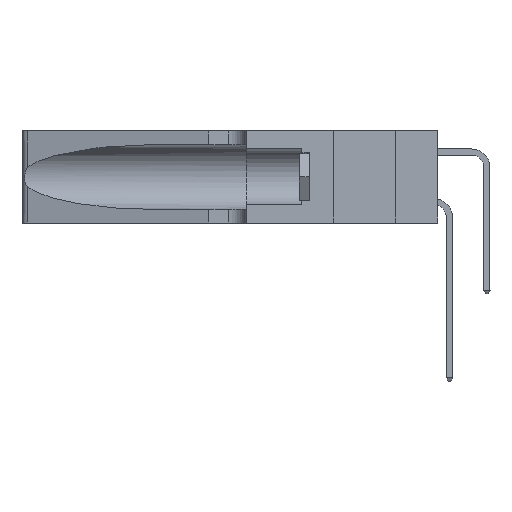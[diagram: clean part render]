
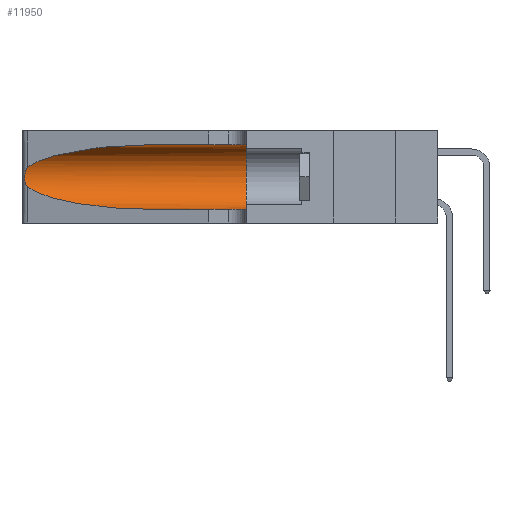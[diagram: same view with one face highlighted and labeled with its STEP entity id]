
A CAD part, left-side view. The second image highlights one B-rep face of the part: STEP entity #11950.
In plain terms, the highlighted cylindrical face has radius 3.308 mm (diameter 6.617 mm), a partial arc.
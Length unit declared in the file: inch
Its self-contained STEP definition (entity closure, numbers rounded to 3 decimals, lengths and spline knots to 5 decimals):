
#690 = CYLINDRICAL_SURFACE ( 'NONE', #15698, 0.13025 ) ;
#820 = CARTESIAN_POINT ( 'NONE',  ( 0.1305, 0.72297, 0.05475 ) ) ;
#1220 = CARTESIAN_POINT ( 'NONE',  ( 0.18966, 0.96281, 0.31525 ) ) ;
#1395 = CARTESIAN_POINT ( 'NONE',  ( 0.25487, 1.22718, 0.22369 ) ) ;
#1634 = EDGE_CURVE ( 'NONE', #3769, #15710, #14663, .T. ) ;
#1723 = CARTESIAN_POINT ( 'NONE',  ( 0.25487, 1.22718, 0.14631 ) ) ;
#2244 = CARTESIAN_POINT ( 'NONE',  ( 0.18966, 0.96281, 0.05475 ) ) ;
#3010 = CARTESIAN_POINT ( 'NONE',  ( 0.26018, 1.23835, 0.19895 ) ) ;
#3198 = CARTESIAN_POINT ( 'NONE',  ( 0.1305, 0.72297, 0.31525 ) ) ;
#3457 = ORIENTED_EDGE ( 'NONE', *, *, #22702, .T. ) ;
#3769 = VERTEX_POINT ( 'NONE', #3198 ) ;
#4048 = CARTESIAN_POINT ( 'NONE',  ( 0.25487, 1.22718, 0.22369 ) ) ;
#4293 = EDGE_LOOP ( 'NONE', ( #13909, #17059, #26115, #3457, #21462, #16241 ) ) ;
#4567 = DIRECTION ( 'NONE',  ( 0., -1., 0. ) ) ;
#5808 = CARTESIAN_POINT ( 'NONE',  ( 0.2373, 1.15595, 0.08982 ) ) ;
#5863 = VERTEX_POINT ( 'NONE', #820 ) ;
#6558 =( BOUNDED_CURVE ( )  B_SPLINE_CURVE ( 3, ( #1723, #5808, #2244, #16350 ),
 .UNSPECIFIED., .F., .F. ) 
 B_SPLINE_CURVE_WITH_KNOTS ( ( 4, 4 ),
 ( 3.44316, 4.71239 ),
 .UNSPECIFIED. ) 
 CURVE ( )  GEOMETRIC_REPRESENTATION_ITEM ( )  RATIONAL_B_SPLINE_CURVE ( ( 1., 0.87, 0.87, 1. ) ) 
 REPRESENTATION_ITEM ( '' )  );
#7334 = CIRCLE ( 'NONE', #14410, 0.13025 ) ;
#7349 = DIRECTION ( 'NONE',  ( 0., 0., 1. ) ) ;
#7541 = CARTESIAN_POINT ( 'NONE',  ( 0.25487, 1.22718, 0.14631 ) ) ;
#9154 = CARTESIAN_POINT ( 'NONE',  ( 0.26017, 1.23833, 0.17102 ) ) ;
#9344 = CARTESIAN_POINT ( 'NONE',  ( 0.26075, 1.23896, 0.19203 ) ) ;
#9787 = DIRECTION ( 'NONE',  ( 0., -1., 0. ) ) ;
#10093 = EDGE_CURVE ( 'NONE', #3769, #18203, #12030, .T. ) ;
#10714 = VERTEX_POINT ( 'NONE', #24264 ) ;
#11950 = ADVANCED_FACE ( 'NONE', ( #21880 ), #690, .F. ) ;
#12030 = LINE ( 'NONE', #18358, #20986 ) ;
#12247 = DIRECTION ( 'NONE',  ( 0., -1., 0. ) ) ;
#13439 = CARTESIAN_POINT ( 'NONE',  ( 0.1305, 0.35, 0.185 ) ) ;
#13536 = EDGE_CURVE ( 'NONE', #15710, #10714, #17473, .T. ) ;
#13671 = CARTESIAN_POINT ( 'NONE',  ( 0.25487, 1.22718, 0.22369 ) ) ;
#13806 = CARTESIAN_POINT ( 'NONE',  ( 0.25789, 1.23486, 0.15765 ) ) ;
#13909 = ORIENTED_EDGE ( 'NONE', *, *, #1634, .T. ) ;
#14410 = AXIS2_PLACEMENT_3D ( 'NONE', #13439, #23691, #7349 ) ;
#14488 = CARTESIAN_POINT ( 'NONE',  ( 0.1305, 1.61858, 0.185 ) ) ;
#14663 =( BOUNDED_CURVE ( )  B_SPLINE_CURVE ( 3, ( #19522, #1220, #19618, #1395 ),
 .UNSPECIFIED., .F., .T. ) 
 B_SPLINE_CURVE_WITH_KNOTS ( ( 4, 4 ),
 ( 1.5708, 2.84003 ),
 .UNSPECIFIED. ) 
 CURVE ( )  GEOMETRIC_REPRESENTATION_ITEM ( )  RATIONAL_B_SPLINE_CURVE ( ( 1., 0.87, 0.87, 1. ) ) 
 REPRESENTATION_ITEM ( '' )  );
#15292 = CARTESIAN_POINT ( 'NONE',  ( 0.25787, 1.23484, 0.2124 ) ) ;
#15698 = AXIS2_PLACEMENT_3D ( 'NONE', #14488, #4567, #18054 ) ;
#15710 = VERTEX_POINT ( 'NONE', #4048 ) ;
#16241 = ORIENTED_EDGE ( 'NONE', *, *, #10093, .F. ) ;
#16350 = CARTESIAN_POINT ( 'NONE',  ( 0.1305, 0.72297, 0.05475 ) ) ;
#16392 = VERTEX_POINT ( 'NONE', #22306 ) ;
#17059 = ORIENTED_EDGE ( 'NONE', *, *, #13536, .T. ) ;
#17473 = B_SPLINE_CURVE_WITH_KNOTS ( 'NONE', 3,
 ( #13671, #19026, #25496, #15292, #19523, #3010, #9344, #21497, #9154, #23539, #13806, #21755, #25934, #7541 ),
 .UNSPECIFIED., .F., .F.,
 ( 4, 2, 2, 2, 2, 2, 4 ),
 ( 0., 0.00027, 0.00053, 0.00107, 0.0016, 0.00187, 0.00214 ),
 .UNSPECIFIED. ) ;
#18054 = DIRECTION ( 'NONE',  ( 0., 0., -1. ) ) ;
#18203 = VERTEX_POINT ( 'NONE', #23053 ) ;
#18358 = CARTESIAN_POINT ( 'NONE',  ( 0.1305, 1.61858, 0.31525 ) ) ;
#19026 = CARTESIAN_POINT ( 'NONE',  ( 0.25555, 1.22994, 0.2215 ) ) ;
#19325 = EDGE_CURVE ( 'NONE', #10714, #5863, #6558, .T. ) ;
#19522 = CARTESIAN_POINT ( 'NONE',  ( 0.1305, 0.72297, 0.31525 ) ) ;
#19523 = CARTESIAN_POINT ( 'NONE',  ( 0.25854, 1.2359, 0.20912 ) ) ;
#19618 = CARTESIAN_POINT ( 'NONE',  ( 0.2373, 1.15595, 0.28018 ) ) ;
#20169 = CARTESIAN_POINT ( 'NONE',  ( 0.1305, 1.61858, 0.05475 ) ) ;
#20567 = LINE ( 'NONE', #20169, #25965 ) ;
#20986 = VECTOR ( 'NONE', #12247, 39.37008 ) ;
#21462 = ORIENTED_EDGE ( 'NONE', *, *, #23250, .F. ) ;
#21497 = CARTESIAN_POINT ( 'NONE',  ( 0.26075, 1.23896, 0.178 ) ) ;
#21755 = CARTESIAN_POINT ( 'NONE',  ( 0.25639, 1.23186, 0.15144 ) ) ;
#21880 = FACE_OUTER_BOUND ( 'NONE', #4293, .T. ) ;
#22306 = CARTESIAN_POINT ( 'NONE',  ( 0.1305, 0.35, 0.05475 ) ) ;
#22702 = EDGE_CURVE ( 'NONE', #5863, #16392, #20567, .T. ) ;
#23053 = CARTESIAN_POINT ( 'NONE',  ( 0.1305, 0.35, 0.31525 ) ) ;
#23250 = EDGE_CURVE ( 'NONE', #18203, #16392, #7334, .T. ) ;
#23539 = CARTESIAN_POINT ( 'NONE',  ( 0.25856, 1.23593, 0.16098 ) ) ;
#23691 = DIRECTION ( 'NONE',  ( 0., 1., 0. ) ) ;
#24264 = CARTESIAN_POINT ( 'NONE',  ( 0.25487, 1.22718, 0.14631 ) ) ;
#25496 = CARTESIAN_POINT ( 'NONE',  ( 0.25639, 1.23184, 0.21858 ) ) ;
#25934 = CARTESIAN_POINT ( 'NONE',  ( 0.25555, 1.22993, 0.14849 ) ) ;
#25965 = VECTOR ( 'NONE', #9787, 39.37008 ) ;
#26115 = ORIENTED_EDGE ( 'NONE', *, *, #19325, .T. ) ;
